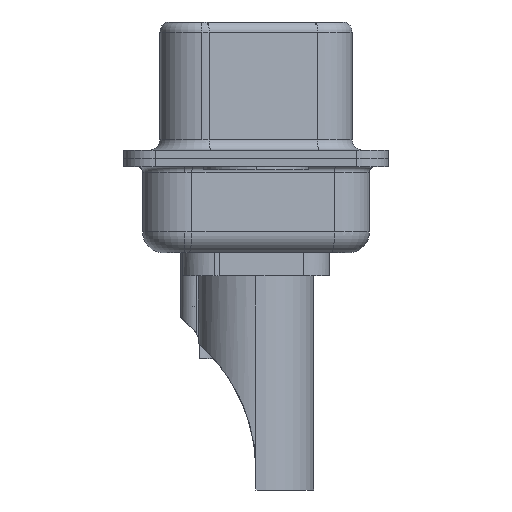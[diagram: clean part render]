
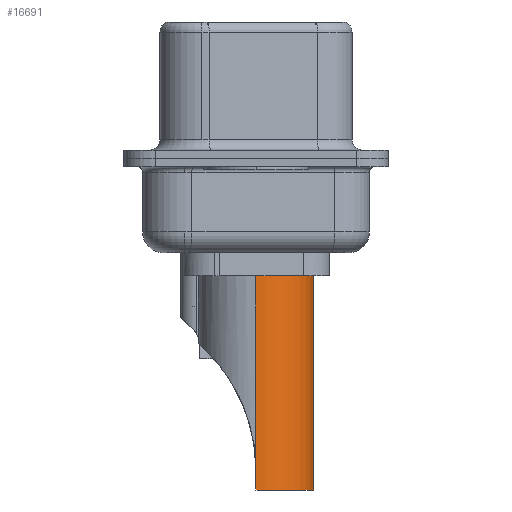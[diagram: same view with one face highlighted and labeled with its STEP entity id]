
A CAD part, left-side view. The second image highlights one B-rep face of the part: STEP entity #16691.
In plain terms, the highlighted cylindrical face has radius 2.75 mm (diameter 5.5 mm), a partial arc.
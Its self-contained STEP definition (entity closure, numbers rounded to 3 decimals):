
#205 = CARTESIAN_POINT ( 'NONE',  ( 2.75, 0., -8.7 ) ) ;
#620 = CARTESIAN_POINT ( 'NONE',  ( 0., 0., 4.234 ) ) ;
#1041 = DIRECTION ( 'NONE',  ( 0., 0., -1. ) ) ;
#1334 = DIRECTION ( 'NONE',  ( 1., 0., 0. ) ) ;
#1406 = CARTESIAN_POINT ( 'NONE',  ( 2.75, 0., -7.764 ) ) ;
#1954 = VECTOR ( 'NONE', #6929, 1000. ) ;
#2703 = CARTESIAN_POINT ( 'NONE',  ( -2.75, 0., 4.234 ) ) ;
#2754 = VERTEX_POINT ( 'NONE', #10600 ) ;
#3079 = CARTESIAN_POINT ( 'NONE',  ( -2.75, 0., -7.764 ) ) ;
#3165 = EDGE_LOOP ( 'NONE', ( #14375, #3953, #4140, #17402, #4024, #9612 ) ) ;
#3518 = DIRECTION ( 'NONE',  ( 0., 0., -1. ) ) ;
#3540 = CIRCLE ( 'NONE', #17504, 2.75 ) ;
#3953 = ORIENTED_EDGE ( 'NONE', *, *, #9565, .T. ) ;
#4024 = ORIENTED_EDGE ( 'NONE', *, *, #6669, .T. ) ;
#4140 = ORIENTED_EDGE ( 'NONE', *, *, #13430, .T. ) ;
#4626 = FACE_OUTER_BOUND ( 'NONE', #3165, .T. ) ;
#4948 = VERTEX_POINT ( 'NONE', #1406 ) ;
#5332 = DIRECTION ( 'NONE',  ( 0., 0., 1. ) ) ;
#5430 = AXIS2_PLACEMENT_3D ( 'NONE', #620, #13623, #6379 ) ;
#5580 = VECTOR ( 'NONE', #3518, 1000. ) ;
#5911 = AXIS2_PLACEMENT_3D ( 'NONE', #14060, #5332, #15529 ) ;
#6011 = VERTEX_POINT ( 'NONE', #3079 ) ;
#6379 = DIRECTION ( 'NONE',  ( 1., 0., 0. ) ) ;
#6520 = EDGE_CURVE ( 'NONE', #4948, #11798, #9331, .T. ) ;
#6669 = EDGE_CURVE ( 'NONE', #4948, #8076, #14461, .T. ) ;
#6929 = DIRECTION ( 'NONE',  ( 0., 0., 1. ) ) ;
#7106 = VECTOR ( 'NONE', #18273, 1000. ) ;
#7310 = CIRCLE ( 'NONE', #5911, 2.75 ) ;
#8076 = VERTEX_POINT ( 'NONE', #17498 ) ;
#8122 = CARTESIAN_POINT ( 'NONE',  ( -2.75, 0., -8.7 ) ) ;
#8506 = EDGE_CURVE ( 'NONE', #6011, #18042, #17856, .T. ) ;
#9331 = LINE ( 'NONE', #205, #5580 ) ;
#9565 = EDGE_CURVE ( 'NONE', #6011, #2754, #16447, .T. ) ;
#9612 = ORIENTED_EDGE ( 'NONE', *, *, #14586, .F. ) ;
#9824 = DIRECTION ( 'NONE',  ( 0., 0., 1. ) ) ;
#10600 = CARTESIAN_POINT ( 'NONE',  ( -2.75, 0., -8.7 ) ) ;
#10896 = CYLINDRICAL_SURFACE ( 'NONE', #5430, 2.75 ) ;
#11798 = VERTEX_POINT ( 'NONE', #11886 ) ;
#11886 = CARTESIAN_POINT ( 'NONE',  ( 2.75, 0., -8.7 ) ) ;
#12380 = CARTESIAN_POINT ( 'NONE',  ( 2.75, 0., 4.234 ) ) ;
#12440 = CARTESIAN_POINT ( 'NONE',  ( -2.75, 0., 1.5 ) ) ;
#13430 = EDGE_CURVE ( 'NONE', #2754, #11798, #3540, .T. ) ;
#13623 = DIRECTION ( 'NONE',  ( 0., 0., 1. ) ) ;
#14060 = CARTESIAN_POINT ( 'NONE',  ( 0., 0., 1.5 ) ) ;
#14375 = ORIENTED_EDGE ( 'NONE', *, *, #8506, .F. ) ;
#14461 = LINE ( 'NONE', #12380, #7106 ) ;
#14586 = EDGE_CURVE ( 'NONE', #18042, #8076, #7310, .T. ) ;
#15504 = VECTOR ( 'NONE', #1041, 1000. ) ;
#15529 = DIRECTION ( 'NONE',  ( 1., 0., 0. ) ) ;
#16447 = LINE ( 'NONE', #8122, #15504 ) ;
#16691 = ADVANCED_FACE ( 'NONE', ( #4626 ), #10896, .T. ) ;
#17402 = ORIENTED_EDGE ( 'NONE', *, *, #6520, .F. ) ;
#17498 = CARTESIAN_POINT ( 'NONE',  ( 2.75, 0., 1.5 ) ) ;
#17504 = AXIS2_PLACEMENT_3D ( 'NONE', #18685, #9824, #1334 ) ;
#17856 = LINE ( 'NONE', #2703, #1954 ) ;
#18042 = VERTEX_POINT ( 'NONE', #12440 ) ;
#18273 = DIRECTION ( 'NONE',  ( 0., 0., 1. ) ) ;
#18685 = CARTESIAN_POINT ( 'NONE',  ( 0., 0., -8.7 ) ) ;
